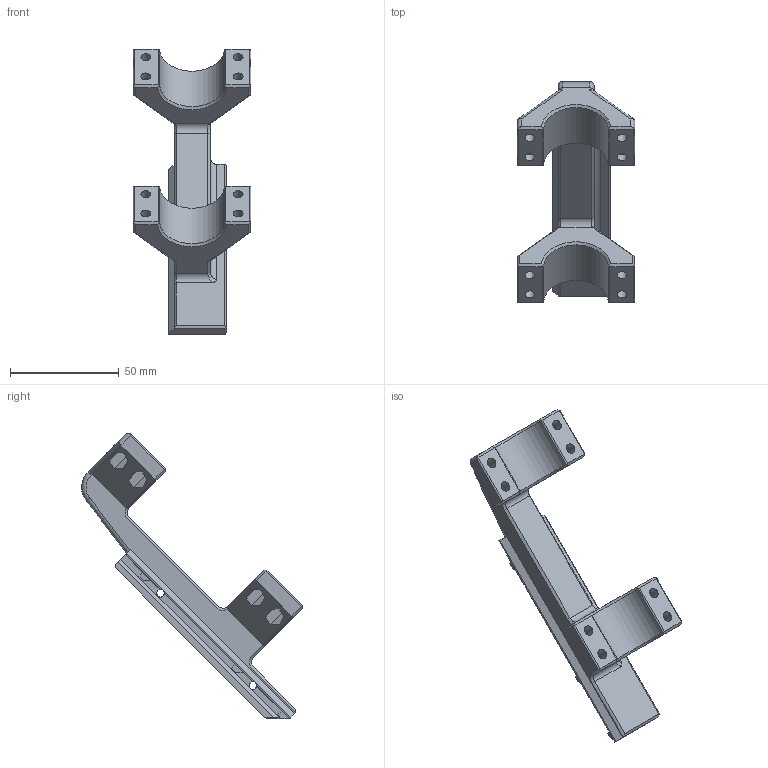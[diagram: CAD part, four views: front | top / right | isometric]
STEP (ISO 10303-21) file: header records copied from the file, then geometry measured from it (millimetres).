
FILE_DESCRIPTION(/* description */ (''),/* implementation_level */ '2;1');
FILE_NAME(/* name */ 'LPL Body - 1.64in.step',/* time_stamp */ '2022-10-10T22:12:51-05:00',/* author */ (''),/* organization */ (''),/* preprocessor_version */ 'ST-DEVELOPER v19',/* originating_system */ 'Autodesk Translation Framework v11.7.0.108',/* authorisation */ '');
FILE_SCHEMA (('AUTOMOTIVE_DESIGN { 1 0 10303 214 3 1 1 }'));
Length unit declared in the file: millimetre
Products named in the file (1): LPL Optic Mount
Bounding box: 54 x 101.36 x 131.24 mm (x, y, z)
Volume: 67994 mm3; surface area: 22553 mm2
Topology: 1 solids, 1 shells, 218 faces, 594 edges, 386 vertices
Faces by surface type: plane 159, cylinder 35, bspline 13, cone 9, torus 2
Full cylindrical faces by diameter (mm): 4.5 x8
Entity records: 7452 total; most frequent: CARTESIAN_POINT 1968, ORIENTED_EDGE 1188, DIRECTION 1029, EDGE_CURVE 594, LINE 451, VECTOR 451, VERTEX_POINT 386, AXIS2_PLACEMENT_3D 289
